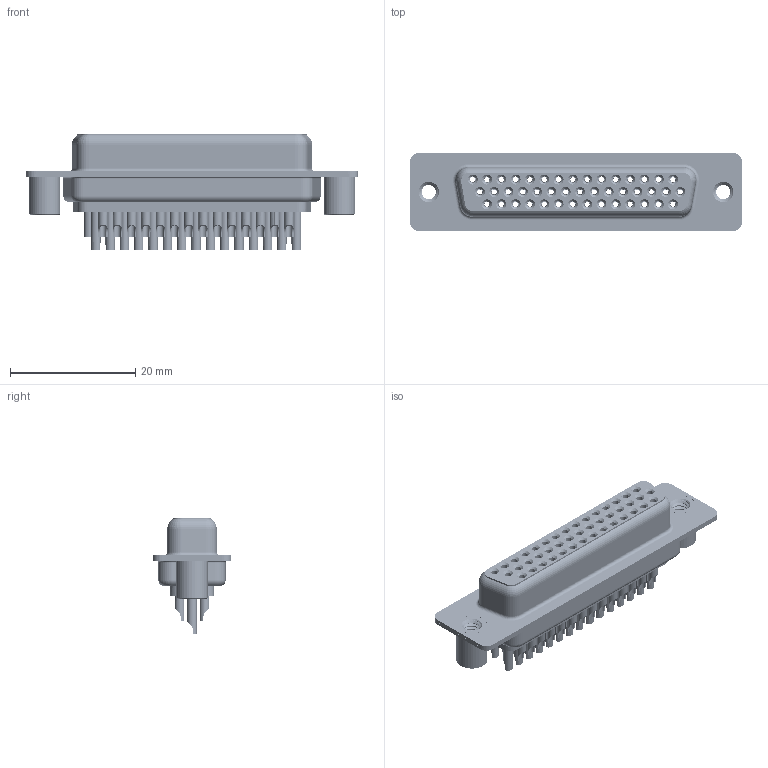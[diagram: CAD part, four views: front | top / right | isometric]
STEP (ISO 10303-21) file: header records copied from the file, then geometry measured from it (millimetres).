
FILE_DESCRIPTION (( 'STEP AP203' ), '1' );
FILE_NAME ('638-044-332-049.STEP', '2020-07-18T23:30:29', ( '' ), ( '' ), 'SwSTEP 2.0', 'SolidWorks 2020', '' );
FILE_SCHEMA (( 'CONFIG_CONTROL_DESIGN' ));
Length unit declared in the file: millimetre
Products named in the file (8): 638-044-332-049; 638 Contact Row 2_32; 638 Shell Rear_44 Contacts; 638 Contact Row 3_32; 638 Shell Front_44 Contacts; 638 4-40 Threaded Standoff BS; 638 Contact Row 1_32; 638 Housing_44 Contacts
Assembly tree (49 placements, depth 2):
  638-044-332-049
    638 Housing_44 Contacts
    638 Shell Front_44 Contacts
    638 Shell Rear_44 Contacts
    638 Contact Row 1_32  x15
    638 Contact Row 2_32  x15
    638 Contact Row 3_32  x14
    638 4-40 Threaded Standoff BS  x2
Bounding box: 53.04 x 12.6 x 18.6 mm (x, y, z)
Volume: 3439.9 mm3; surface area: 13716.6 mm2
Topology: 49 solids, 49 shells, 4217 faces, 10693 edges, 6717 vertices
Faces by surface type: cylinder 1257, plane 991, bspline 886, torus 849, cone 234
Entity records: 36609 total; most frequent: CARTESIAN_POINT 9912, DIRECTION 5496, ORIENTED_EDGE 4924, EDGE_CURVE 2462, AXIS2_PLACEMENT_3D 2316, VERTEX_POINT 1560, EDGE_LOOP 1300, CIRCLE 1270
